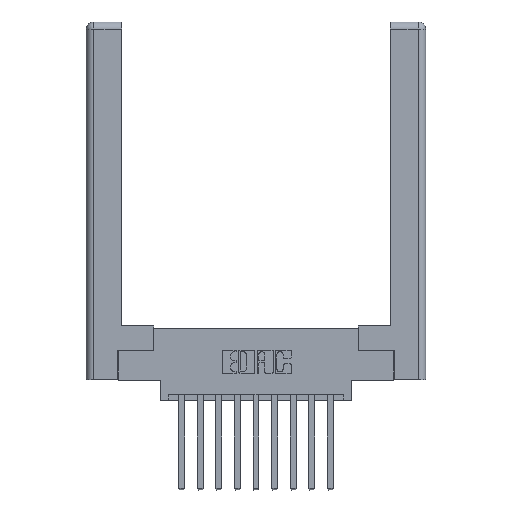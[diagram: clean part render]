
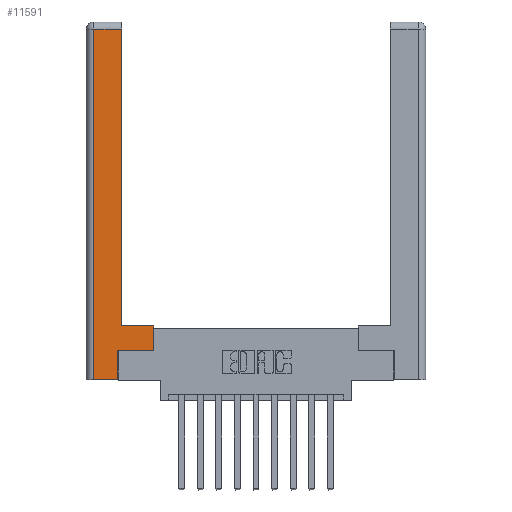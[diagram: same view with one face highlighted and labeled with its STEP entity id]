
A CAD part, top view. The second image highlights one B-rep face of the part: STEP entity #11591.
In plain terms, the highlighted planar face has unit normal (0, 0, 1).
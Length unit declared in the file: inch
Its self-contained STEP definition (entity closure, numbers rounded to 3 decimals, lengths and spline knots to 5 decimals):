
#10 = LINE ( 'NONE', #4741, #5528 ) ;
#261 = DIRECTION ( 'NONE',  ( 0., 1., 0. ) ) ;
#411 = VERTEX_POINT ( 'NONE', #2753 ) ;
#563 = DIRECTION ( 'NONE',  ( -1., 0., 0. ) ) ;
#636 = CARTESIAN_POINT ( 'NONE',  ( 0.265, 0.245, 0. ) ) ;
#1220 = VERTEX_POINT ( 'NONE', #2485 ) ;
#1353 = CARTESIAN_POINT ( 'NONE',  ( 0., 0., 0. ) ) ;
#1385 = EDGE_CURVE ( 'NONE', #411, #11602, #11250, .T. ) ;
#1584 = DIRECTION ( 'NONE',  ( 0., 1., 0. ) ) ;
#1838 = VECTOR ( 'NONE', #261, 39.37008 ) ;
#2339 = ORIENTED_EDGE ( 'NONE', *, *, #10748, .T. ) ;
#2485 = CARTESIAN_POINT ( 'NONE',  ( 0.265, 0.245, 0. ) ) ;
#2571 = DIRECTION ( 'NONE',  ( -1., 0., 0. ) ) ;
#2753 = CARTESIAN_POINT ( 'NONE',  ( 0.295, 0.45, 0. ) ) ;
#2817 = CARTESIAN_POINT ( 'NONE',  ( 0.0615, 2.94, 0. ) ) ;
#2940 = CARTESIAN_POINT ( 'NONE',  ( 0.0615, 0., 0. ) ) ;
#3210 = EDGE_CURVE ( 'NONE', #8483, #411, #4049, .T. ) ;
#3310 = CARTESIAN_POINT ( 'NONE',  ( 0.0615, 0., 0. ) ) ;
#3383 = EDGE_CURVE ( 'NONE', #9233, #8483, #8929, .T. ) ;
#3503 = LINE ( 'NONE', #5105, #7398 ) ;
#3616 = PLANE ( 'NONE',  #4990 ) ;
#4049 = LINE ( 'NONE', #6708, #7111 ) ;
#4075 = CARTESIAN_POINT ( 'NONE',  ( 0.565, 0.45, 0. ) ) ;
#4188 = VERTEX_POINT ( 'NONE', #2940 ) ;
#4447 = ORIENTED_EDGE ( 'NONE', *, *, #1385, .T. ) ;
#4712 = DIRECTION ( 'NONE',  ( -1., 0., 0. ) ) ;
#4741 = CARTESIAN_POINT ( 'NONE',  ( 0.0615, 2.94, 0. ) ) ;
#4797 = ORIENTED_EDGE ( 'NONE', *, *, #10580, .T. ) ;
#4915 = VECTOR ( 'NONE', #12367, 39.37008 ) ;
#4990 = AXIS2_PLACEMENT_3D ( 'NONE', #1353, #10089, #2571 ) ;
#5105 = CARTESIAN_POINT ( 'NONE',  ( 0.565, 0.245, 0. ) ) ;
#5528 = VECTOR ( 'NONE', #563, 39.37008 ) ;
#6676 = EDGE_LOOP ( 'NONE', ( #4447, #2339, #13507, #7650, #9656, #4797, #13340, #12779 ) ) ;
#6708 = CARTESIAN_POINT ( 'NONE',  ( 0.295, 0.45, 0. ) ) ;
#7111 = VECTOR ( 'NONE', #4712, 39.37008 ) ;
#7163 = VECTOR ( 'NONE', #10850, 39.37008 ) ;
#7398 = VECTOR ( 'NONE', #10693, 39.37008 ) ;
#7650 = ORIENTED_EDGE ( 'NONE', *, *, #13285, .T. ) ;
#7678 = CARTESIAN_POINT ( 'NONE',  ( 0.265, 0., 0. ) ) ;
#7759 = VECTOR ( 'NONE', #1584, 39.37008 ) ;
#7792 = LINE ( 'NONE', #9251, #4915 ) ;
#8348 = EDGE_CURVE ( 'NONE', #13738, #1220, #10603, .T. ) ;
#8475 = FACE_OUTER_BOUND ( 'NONE', #6676, .T. ) ;
#8483 = VERTEX_POINT ( 'NONE', #4075 ) ;
#8832 = LINE ( 'NONE', #3310, #7163 ) ;
#8929 = LINE ( 'NONE', #9121, #7759 ) ;
#8982 = DIRECTION ( 'NONE',  ( 0., 1., 0. ) ) ;
#9023 = CARTESIAN_POINT ( 'NONE',  ( 0.295, 2.94, 0. ) ) ;
#9121 = CARTESIAN_POINT ( 'NONE',  ( 0.565, 0.45, 0. ) ) ;
#9233 = VERTEX_POINT ( 'NONE', #9494 ) ;
#9251 = CARTESIAN_POINT ( 'NONE',  ( 0.265, 0., 0. ) ) ;
#9494 = CARTESIAN_POINT ( 'NONE',  ( 0.565, 0.245, 0. ) ) ;
#9656 = ORIENTED_EDGE ( 'NONE', *, *, #8348, .T. ) ;
#10089 = DIRECTION ( 'NONE',  ( 0., 0., -1. ) ) ;
#10580 = EDGE_CURVE ( 'NONE', #1220, #9233, #3503, .T. ) ;
#10603 = LINE ( 'NONE', #636, #12753 ) ;
#10693 = DIRECTION ( 'NONE',  ( 1., 0., 0. ) ) ;
#10748 = EDGE_CURVE ( 'NONE', #11602, #10926, #10, .T. ) ;
#10850 = DIRECTION ( 'NONE',  ( 0., -1., 0. ) ) ;
#10926 = VERTEX_POINT ( 'NONE', #2817 ) ;
#11250 = LINE ( 'NONE', #12118, #1838 ) ;
#11591 = ADVANCED_FACE ( 'NONE', ( #8475 ), #3616, .F. ) ;
#11602 = VERTEX_POINT ( 'NONE', #9023 ) ;
#11768 = EDGE_CURVE ( 'NONE', #10926, #4188, #8832, .T. ) ;
#12118 = CARTESIAN_POINT ( 'NONE',  ( 0.295, 3., 0. ) ) ;
#12367 = DIRECTION ( 'NONE',  ( 1., 0., 0. ) ) ;
#12753 = VECTOR ( 'NONE', #8982, 39.37008 ) ;
#12779 = ORIENTED_EDGE ( 'NONE', *, *, #3210, .T. ) ;
#13285 = EDGE_CURVE ( 'NONE', #4188, #13738, #7792, .T. ) ;
#13340 = ORIENTED_EDGE ( 'NONE', *, *, #3383, .T. ) ;
#13507 = ORIENTED_EDGE ( 'NONE', *, *, #11768, .T. ) ;
#13738 = VERTEX_POINT ( 'NONE', #7678 ) ;
